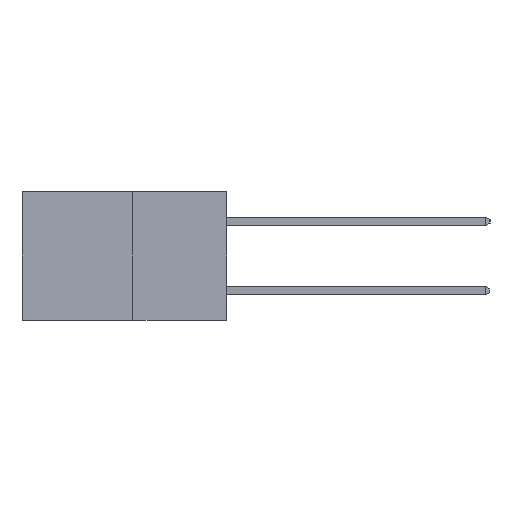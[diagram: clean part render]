
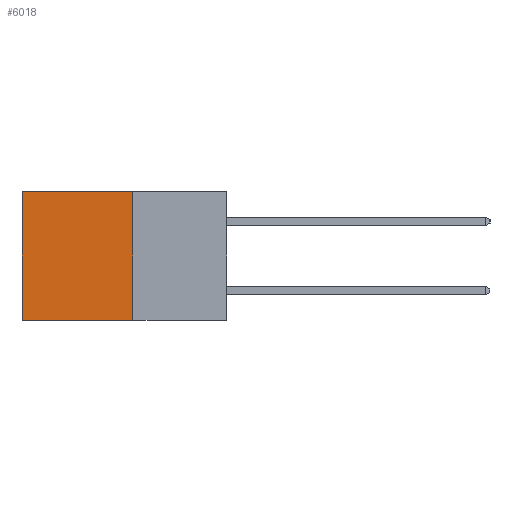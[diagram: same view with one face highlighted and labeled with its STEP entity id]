
A CAD part, left-side view. The second image highlights one B-rep face of the part: STEP entity #6018.
In plain terms, the highlighted planar face has unit normal (-1, 0, 0).
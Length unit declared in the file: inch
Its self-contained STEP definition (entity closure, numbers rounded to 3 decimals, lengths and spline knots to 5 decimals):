
#1150 = DIRECTION ( 'NONE',  ( 0., 0., -1. ) ) ;
#2212 = CARTESIAN_POINT ( 'NONE',  ( 0.277, 0.59, -0.37 ) ) ;
#2429 = EDGE_LOOP ( 'NONE', ( #20480, #2462, #6777, #3497 ) ) ;
#2462 = ORIENTED_EDGE ( 'NONE', *, *, #5259, .F. ) ;
#2537 = LINE ( 'NONE', #20930, #15908 ) ;
#3497 = ORIENTED_EDGE ( 'NONE', *, *, #4118, .T. ) ;
#4118 = EDGE_CURVE ( 'NONE', #4752, #14549, #11559, .T. ) ;
#4616 = EDGE_CURVE ( 'NONE', #14549, #16526, #19170, .T. ) ;
#4752 = VERTEX_POINT ( 'NONE', #21281 ) ;
#5259 = EDGE_CURVE ( 'NONE', #13596, #16526, #2537, .T. ) ;
#6018 = ADVANCED_FACE ( 'NONE', ( #18904 ), #20905, .F. ) ;
#6777 = ORIENTED_EDGE ( 'NONE', *, *, #18525, .F. ) ;
#7050 = VECTOR ( 'NONE', #18411, 39.37008 ) ;
#7343 = CARTESIAN_POINT ( 'NONE',  ( 0.277, 0.27, -0.37 ) ) ;
#7845 = DIRECTION ( 'NONE',  ( 0., 0., -1. ) ) ;
#8964 = CARTESIAN_POINT ( 'NONE',  ( 0.277, 0.59, 0. ) ) ;
#9520 = CARTESIAN_POINT ( 'NONE',  ( 0.277, 0.27, -0.37 ) ) ;
#9544 = DIRECTION ( 'NONE',  ( 0., 1., 0. ) ) ;
#11559 = LINE ( 'NONE', #18391, #7050 ) ;
#11633 = VECTOR ( 'NONE', #17279, 39.37008 ) ;
#13596 = VERTEX_POINT ( 'NONE', #15102 ) ;
#14549 = VERTEX_POINT ( 'NONE', #8964 ) ;
#15102 = CARTESIAN_POINT ( 'NONE',  ( 0.277, 0.27, -0.37 ) ) ;
#15908 = VECTOR ( 'NONE', #9544, 39.37008 ) ;
#16480 = AXIS2_PLACEMENT_3D ( 'NONE', #9520, #17767, #7845 ) ;
#16489 = LINE ( 'NONE', #7343, #11633 ) ;
#16526 = VERTEX_POINT ( 'NONE', #17089 ) ;
#17089 = CARTESIAN_POINT ( 'NONE',  ( 0.277, 0.59, -0.37 ) ) ;
#17279 = DIRECTION ( 'NONE',  ( 0., 0., -1. ) ) ;
#17767 = DIRECTION ( 'NONE',  ( 1., 0., 0. ) ) ;
#18391 = CARTESIAN_POINT ( 'NONE',  ( 0.277, 0.27, 0. ) ) ;
#18411 = DIRECTION ( 'NONE',  ( 0., 1., 0. ) ) ;
#18525 = EDGE_CURVE ( 'NONE', #4752, #13596, #16489, .T. ) ;
#18663 = VECTOR ( 'NONE', #1150, 39.37008 ) ;
#18904 = FACE_OUTER_BOUND ( 'NONE', #2429, .T. ) ;
#19170 = LINE ( 'NONE', #2212, #18663 ) ;
#20480 = ORIENTED_EDGE ( 'NONE', *, *, #4616, .T. ) ;
#20905 = PLANE ( 'NONE',  #16480 ) ;
#20930 = CARTESIAN_POINT ( 'NONE',  ( 0.277, 0.27, -0.37 ) ) ;
#21281 = CARTESIAN_POINT ( 'NONE',  ( 0.277, 0.27, 0. ) ) ;
